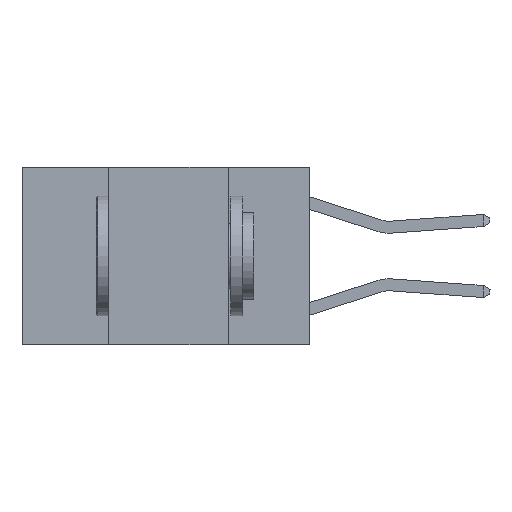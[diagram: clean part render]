
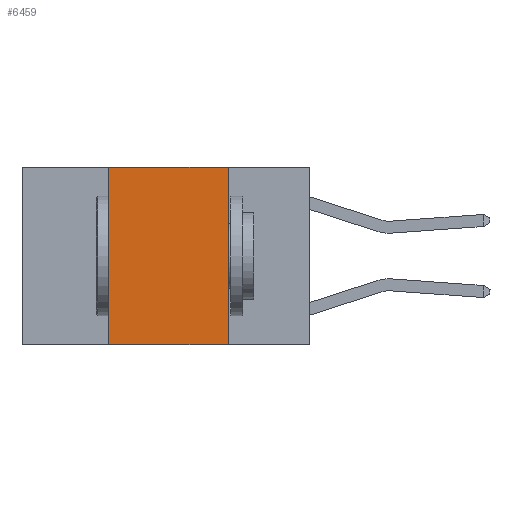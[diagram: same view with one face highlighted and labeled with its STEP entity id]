
A CAD part, left-side view. The second image highlights one B-rep face of the part: STEP entity #6459.
In plain terms, the highlighted planar face has unit normal (-1, 0, 0).
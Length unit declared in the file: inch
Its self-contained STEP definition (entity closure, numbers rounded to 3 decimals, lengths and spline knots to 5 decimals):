
#166 = FACE_OUTER_BOUND ( 'NONE', #7475, .T. ) ;
#804 = LINE ( 'NONE', #900, #978 ) ;
#900 = CARTESIAN_POINT ( 'NONE',  ( 0., 0.42, 0. ) ) ;
#978 = VECTOR ( 'NONE', #2334, 39.37008 ) ;
#1297 = CARTESIAN_POINT ( 'NONE',  ( 0., 0.17, 0. ) ) ;
#1303 = CARTESIAN_POINT ( 'NONE',  ( 0., 0.17, 0. ) ) ;
#1346 = DIRECTION ( 'NONE',  ( 0., 0., -1. ) ) ;
#1661 = ORIENTED_EDGE ( 'NONE', *, *, #4578, .T. ) ;
#2076 = VERTEX_POINT ( 'NONE', #5597 ) ;
#2334 = DIRECTION ( 'NONE',  ( 0., 0., 1. ) ) ;
#2515 = VERTEX_POINT ( 'NONE', #5915 ) ;
#2731 = EDGE_CURVE ( 'NONE', #5960, #2076, #804, .T. ) ;
#3107 = DIRECTION ( 'NONE',  ( 0., 0., -1. ) ) ;
#3308 = EDGE_CURVE ( 'NONE', #2076, #5046, #5009, .T. ) ;
#3720 = LINE ( 'NONE', #7540, #5655 ) ;
#4333 = VECTOR ( 'NONE', #1346, 39.37008 ) ;
#4455 = DIRECTION ( 'NONE',  ( 0., -1., 0. ) ) ;
#4578 = EDGE_CURVE ( 'NONE', #5960, #2515, #3720, .T. ) ;
#4833 = ORIENTED_EDGE ( 'NONE', *, *, #3308, .F. ) ;
#5009 = LINE ( 'NONE', #5790, #7831 ) ;
#5046 = VERTEX_POINT ( 'NONE', #1297 ) ;
#5082 = CARTESIAN_POINT ( 'NONE',  ( 0., 0.42, -0.37 ) ) ;
#5597 = CARTESIAN_POINT ( 'NONE',  ( 0., 0.42, 0. ) ) ;
#5655 = VECTOR ( 'NONE', #4455, 39.37008 ) ;
#5696 = DIRECTION ( 'NONE',  ( 0., -1., 0. ) ) ;
#5790 = CARTESIAN_POINT ( 'NONE',  ( 0., 0.6, 0. ) ) ;
#5915 = CARTESIAN_POINT ( 'NONE',  ( 0., 0.17, -0.37 ) ) ;
#5960 = VERTEX_POINT ( 'NONE', #5082 ) ;
#5976 = CARTESIAN_POINT ( 'NONE',  ( 0., 0.6, 0. ) ) ;
#6459 = ADVANCED_FACE ( 'NONE', ( #166 ), #6713, .F. ) ;
#6713 = PLANE ( 'NONE',  #6943 ) ;
#6854 = DIRECTION ( 'NONE',  ( 1., 0., 0. ) ) ;
#6943 = AXIS2_PLACEMENT_3D ( 'NONE', #5976, #6854, #3107 ) ;
#7475 = EDGE_LOOP ( 'NONE', ( #8144, #4833, #9389, #1661 ) ) ;
#7540 = CARTESIAN_POINT ( 'NONE',  ( 0., 0.6, -0.37 ) ) ;
#7645 = EDGE_CURVE ( 'NONE', #5046, #2515, #7971, .T. ) ;
#7831 = VECTOR ( 'NONE', #5696, 39.37008 ) ;
#7971 = LINE ( 'NONE', #1303, #4333 ) ;
#8144 = ORIENTED_EDGE ( 'NONE', *, *, #7645, .F. ) ;
#9389 = ORIENTED_EDGE ( 'NONE', *, *, #2731, .F. ) ;
